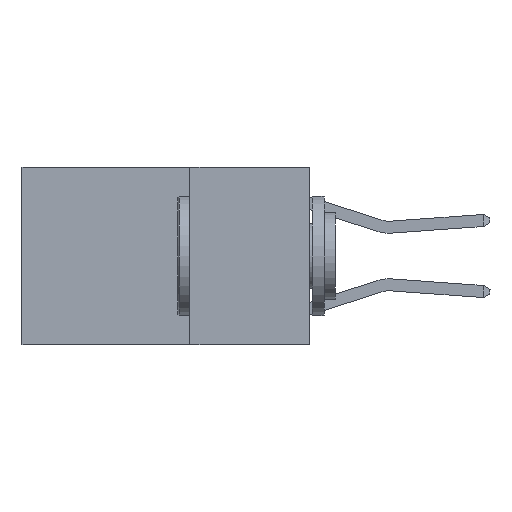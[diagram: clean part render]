
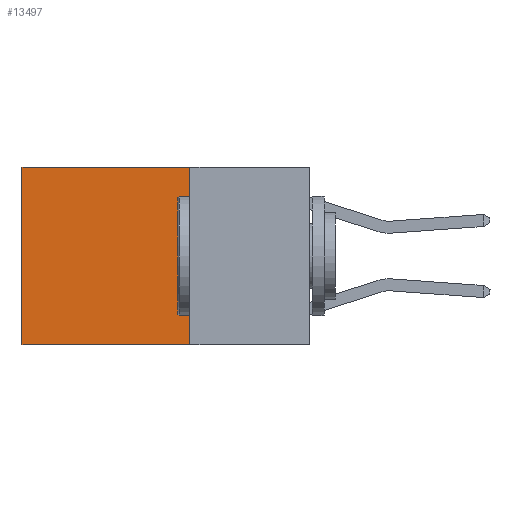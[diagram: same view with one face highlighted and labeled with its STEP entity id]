
A CAD part, left-side view. The second image highlights one B-rep face of the part: STEP entity #13497.
In plain terms, the highlighted planar face has unit normal (-1, 0, 0).
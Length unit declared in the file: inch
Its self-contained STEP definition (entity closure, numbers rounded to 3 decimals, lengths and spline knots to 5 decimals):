
#926 = LINE ( 'NONE', #1223, #4948 ) ;
#1223 = CARTESIAN_POINT ( 'NONE',  ( 0.2625, 0.6, 0. ) ) ;
#1634 = DIRECTION ( 'NONE',  ( 0., 0., -1. ) ) ;
#2850 = ORIENTED_EDGE ( 'NONE', *, *, #14027, .T. ) ;
#3377 = ORIENTED_EDGE ( 'NONE', *, *, #6569, .F. ) ;
#3449 = CARTESIAN_POINT ( 'NONE',  ( 0.2625, 0.25, 0. ) ) ;
#3691 = VECTOR ( 'NONE', #8880, 39.37008 ) ;
#3970 = VECTOR ( 'NONE', #4876, 39.37008 ) ;
#4305 = LINE ( 'NONE', #3449, #8322 ) ;
#4348 = CARTESIAN_POINT ( 'NONE',  ( 0.2625, 0.6, -0.37 ) ) ;
#4829 = VERTEX_POINT ( 'NONE', #4348 ) ;
#4876 = DIRECTION ( 'NONE',  ( 0., 1., 0. ) ) ;
#4948 = VECTOR ( 'NONE', #13166, 39.37008 ) ;
#5200 = DIRECTION ( 'NONE',  ( 0., 0., -1. ) ) ;
#6455 = VERTEX_POINT ( 'NONE', #16764 ) ;
#6569 = EDGE_CURVE ( 'NONE', #17086, #10979, #4305, .T. ) ;
#6887 = AXIS2_PLACEMENT_3D ( 'NONE', #16888, #11842, #1634 ) ;
#7161 = CARTESIAN_POINT ( 'NONE',  ( 0.2625, 0.25, 0. ) ) ;
#7711 = LINE ( 'NONE', #7161, #3691 ) ;
#8322 = VECTOR ( 'NONE', #5200, 39.37008 ) ;
#8880 = DIRECTION ( 'NONE',  ( 0., 1., 0. ) ) ;
#9031 = LINE ( 'NONE', #9913, #3970 ) ;
#9913 = CARTESIAN_POINT ( 'NONE',  ( 0.2625, 0.25, -0.37 ) ) ;
#10127 = PLANE ( 'NONE',  #6887 ) ;
#10979 = VERTEX_POINT ( 'NONE', #18805 ) ;
#11842 = DIRECTION ( 'NONE',  ( 1., 0., 0. ) ) ;
#12990 = ORIENTED_EDGE ( 'NONE', *, *, #17555, .F. ) ;
#13166 = DIRECTION ( 'NONE',  ( 0., 0., -1. ) ) ;
#13497 = ADVANCED_FACE ( 'NONE', ( #15046 ), #10127, .F. ) ;
#14027 = EDGE_CURVE ( 'NONE', #6455, #4829, #926, .T. ) ;
#14854 = CARTESIAN_POINT ( 'NONE',  ( 0.2625, 0.25, 0. ) ) ;
#15046 = FACE_OUTER_BOUND ( 'NONE', #21739, .T. ) ;
#16764 = CARTESIAN_POINT ( 'NONE',  ( 0.2625, 0.6, 0. ) ) ;
#16888 = CARTESIAN_POINT ( 'NONE',  ( 0.2625, 0.25, 0. ) ) ;
#17086 = VERTEX_POINT ( 'NONE', #14854 ) ;
#17555 = EDGE_CURVE ( 'NONE', #10979, #4829, #9031, .T. ) ;
#17811 = EDGE_CURVE ( 'NONE', #17086, #6455, #7711, .T. ) ;
#17879 = ORIENTED_EDGE ( 'NONE', *, *, #17811, .T. ) ;
#18805 = CARTESIAN_POINT ( 'NONE',  ( 0.2625, 0.25, -0.37 ) ) ;
#21739 = EDGE_LOOP ( 'NONE', ( #2850, #12990, #3377, #17879 ) ) ;
